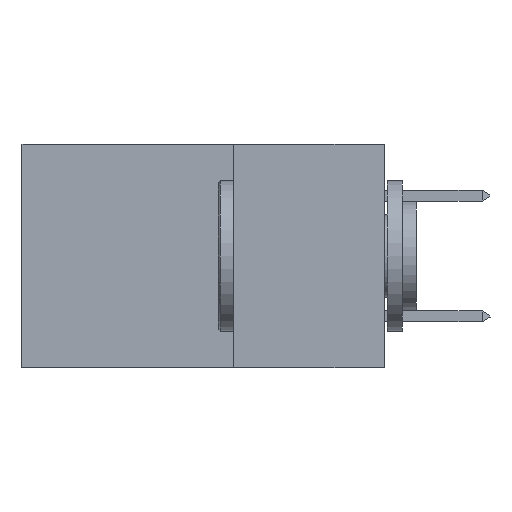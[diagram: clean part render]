
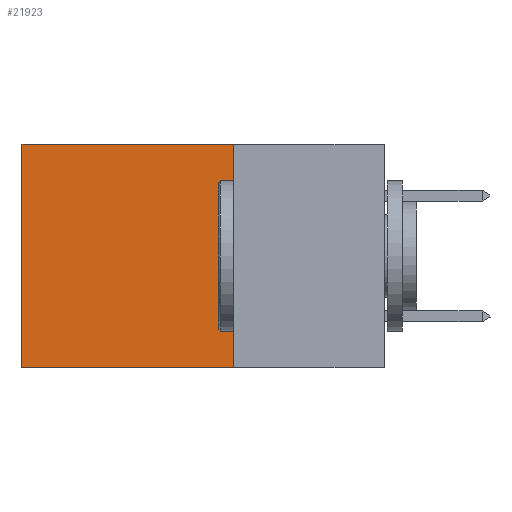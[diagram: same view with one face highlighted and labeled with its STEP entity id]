
A CAD part, left-side view. The second image highlights one B-rep face of the part: STEP entity #21923.
In plain terms, the highlighted planar face has unit normal (-1, 0, 0).
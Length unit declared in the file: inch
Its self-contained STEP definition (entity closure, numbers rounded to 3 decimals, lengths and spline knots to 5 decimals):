
#534 = VERTEX_POINT ( 'NONE', #18108 ) ;
#1142 = PLANE ( 'NONE',  #8120 ) ;
#3390 = CARTESIAN_POINT ( 'NONE',  ( 0.2875, 0.6, -0.37 ) ) ;
#3902 = CARTESIAN_POINT ( 'NONE',  ( 0.2875, 0.25, 0. ) ) ;
#4329 = EDGE_CURVE ( 'NONE', #534, #27137, #7905, .T. ) ;
#5516 = CARTESIAN_POINT ( 'NONE',  ( 0.2875, 0.6, 0. ) ) ;
#7130 = VECTOR ( 'NONE', #25188, 39.37008 ) ;
#7334 = DIRECTION ( 'NONE',  ( 0., 0., -1. ) ) ;
#7904 = EDGE_LOOP ( 'NONE', ( #11646, #16798, #8482, #23363 ) ) ;
#7905 = LINE ( 'NONE', #13785, #14738 ) ;
#7907 = DIRECTION ( 'NONE',  ( 1., 0., 0. ) ) ;
#8120 = AXIS2_PLACEMENT_3D ( 'NONE', #3902, #7907, #12348 ) ;
#8197 = LINE ( 'NONE', #13822, #11947 ) ;
#8482 = ORIENTED_EDGE ( 'NONE', *, *, #4329, .F. ) ;
#8508 = VECTOR ( 'NONE', #20928, 39.37008 ) ;
#10096 = CARTESIAN_POINT ( 'NONE',  ( 0.2875, 0.25, 0. ) ) ;
#11646 = ORIENTED_EDGE ( 'NONE', *, *, #13006, .T. ) ;
#11947 = VECTOR ( 'NONE', #27046, 39.37008 ) ;
#12348 = DIRECTION ( 'NONE',  ( 0., 0., -1. ) ) ;
#12756 = CARTESIAN_POINT ( 'NONE',  ( 0.2875, 0.25, -0.37 ) ) ;
#13006 = EDGE_CURVE ( 'NONE', #21263, #17806, #8197, .T. ) ;
#13785 = CARTESIAN_POINT ( 'NONE',  ( 0.2875, 0.25, 0. ) ) ;
#13822 = CARTESIAN_POINT ( 'NONE',  ( 0.2875, 0.6, 0. ) ) ;
#14738 = VECTOR ( 'NONE', #7334, 39.37008 ) ;
#15172 = CARTESIAN_POINT ( 'NONE',  ( 0.2875, 0.25, -0.37 ) ) ;
#16798 = ORIENTED_EDGE ( 'NONE', *, *, #22483, .F. ) ;
#16821 = EDGE_CURVE ( 'NONE', #534, #21263, #24351, .T. ) ;
#17806 = VERTEX_POINT ( 'NONE', #3390 ) ;
#18108 = CARTESIAN_POINT ( 'NONE',  ( 0.2875, 0.25, 0. ) ) ;
#20079 = FACE_OUTER_BOUND ( 'NONE', #7904, .T. ) ;
#20928 = DIRECTION ( 'NONE',  ( 0., 1., 0. ) ) ;
#21263 = VERTEX_POINT ( 'NONE', #5516 ) ;
#21923 = ADVANCED_FACE ( 'NONE', ( #20079 ), #1142, .F. ) ;
#22483 = EDGE_CURVE ( 'NONE', #27137, #17806, #27708, .T. ) ;
#23363 = ORIENTED_EDGE ( 'NONE', *, *, #16821, .T. ) ;
#24351 = LINE ( 'NONE', #10096, #7130 ) ;
#25188 = DIRECTION ( 'NONE',  ( 0., 1., 0. ) ) ;
#27046 = DIRECTION ( 'NONE',  ( 0., 0., -1. ) ) ;
#27137 = VERTEX_POINT ( 'NONE', #12756 ) ;
#27708 = LINE ( 'NONE', #15172, #8508 ) ;
